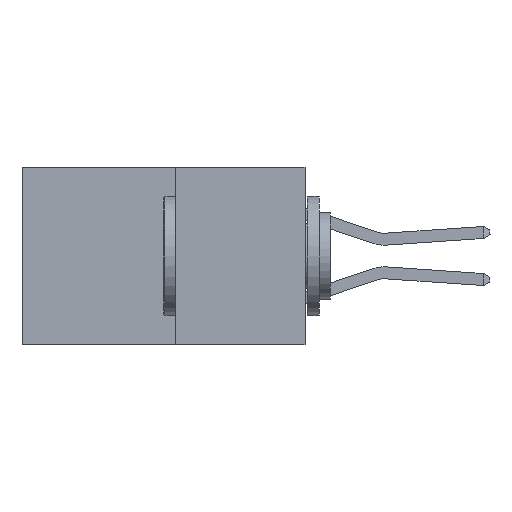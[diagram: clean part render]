
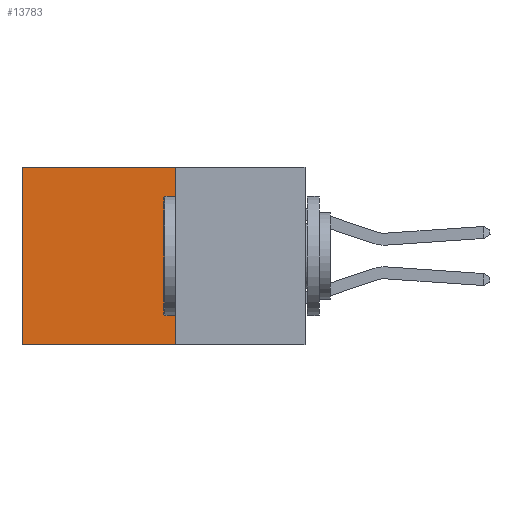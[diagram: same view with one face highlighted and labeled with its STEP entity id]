
A CAD part, left-side view. The second image highlights one B-rep face of the part: STEP entity #13783.
In plain terms, the highlighted planar face has unit normal (-1, 0, 0).
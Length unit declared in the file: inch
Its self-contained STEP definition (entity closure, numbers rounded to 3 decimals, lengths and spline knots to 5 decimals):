
#268 = VERTEX_POINT ( 'NONE', #6615 ) ;
#974 = EDGE_CURVE ( 'NONE', #24079, #268, #27560, .T. ) ;
#3010 = LINE ( 'NONE', #26014, #19341 ) ;
#5241 = VERTEX_POINT ( 'NONE', #17669 ) ;
#5438 = ORIENTED_EDGE ( 'NONE', *, *, #23254, .T. ) ;
#6615 = CARTESIAN_POINT ( 'NONE',  ( 0.277, 0.59, 0. ) ) ;
#7890 = ORIENTED_EDGE ( 'NONE', *, *, #9038, .F. ) ;
#8226 = ORIENTED_EDGE ( 'NONE', *, *, #22736, .F. ) ;
#8576 = CARTESIAN_POINT ( 'NONE',  ( 0.277, 0.27, 0. ) ) ;
#8924 = DIRECTION ( 'NONE',  ( 0., 1., 0. ) ) ;
#9038 = EDGE_CURVE ( 'NONE', #24079, #27092, #23679, .T. ) ;
#9127 = EDGE_LOOP ( 'NONE', ( #5438, #8226, #7890, #14503 ) ) ;
#10034 = CARTESIAN_POINT ( 'NONE',  ( 0.277, 0.27, -0.37 ) ) ;
#10278 = DIRECTION ( 'NONE',  ( 0., 0., -1. ) ) ;
#11430 = AXIS2_PLACEMENT_3D ( 'NONE', #21241, #23551, #10278 ) ;
#13306 = CARTESIAN_POINT ( 'NONE',  ( 0.277, 0.27, 0. ) ) ;
#13783 = ADVANCED_FACE ( 'NONE', ( #25291 ), #21337, .F. ) ;
#14503 = ORIENTED_EDGE ( 'NONE', *, *, #974, .T. ) ;
#15574 = CARTESIAN_POINT ( 'NONE',  ( 0.277, 0.27, -0.37 ) ) ;
#17669 = CARTESIAN_POINT ( 'NONE',  ( 0.277, 0.59, -0.37 ) ) ;
#17831 = VECTOR ( 'NONE', #27674, 39.37008 ) ;
#19341 = VECTOR ( 'NONE', #28144, 39.37008 ) ;
#20380 = VECTOR ( 'NONE', #28519, 39.37008 ) ;
#21241 = CARTESIAN_POINT ( 'NONE',  ( 0.277, 0.27, -0.37 ) ) ;
#21337 = PLANE ( 'NONE',  #11430 ) ;
#21442 = LINE ( 'NONE', #22198, #27910 ) ;
#22198 = CARTESIAN_POINT ( 'NONE',  ( 0.277, 0.27, -0.37 ) ) ;
#22736 = EDGE_CURVE ( 'NONE', #27092, #5241, #21442, .T. ) ;
#23254 = EDGE_CURVE ( 'NONE', #268, #5241, #3010, .T. ) ;
#23551 = DIRECTION ( 'NONE',  ( 1., 0., 0. ) ) ;
#23679 = LINE ( 'NONE', #10034, #17831 ) ;
#24079 = VERTEX_POINT ( 'NONE', #8576 ) ;
#25291 = FACE_OUTER_BOUND ( 'NONE', #9127, .T. ) ;
#26014 = CARTESIAN_POINT ( 'NONE',  ( 0.277, 0.59, -0.37 ) ) ;
#27092 = VERTEX_POINT ( 'NONE', #15574 ) ;
#27560 = LINE ( 'NONE', #13306, #20380 ) ;
#27674 = DIRECTION ( 'NONE',  ( 0., 0., -1. ) ) ;
#27910 = VECTOR ( 'NONE', #8924, 39.37008 ) ;
#28144 = DIRECTION ( 'NONE',  ( 0., 0., -1. ) ) ;
#28519 = DIRECTION ( 'NONE',  ( 0., 1., 0. ) ) ;
